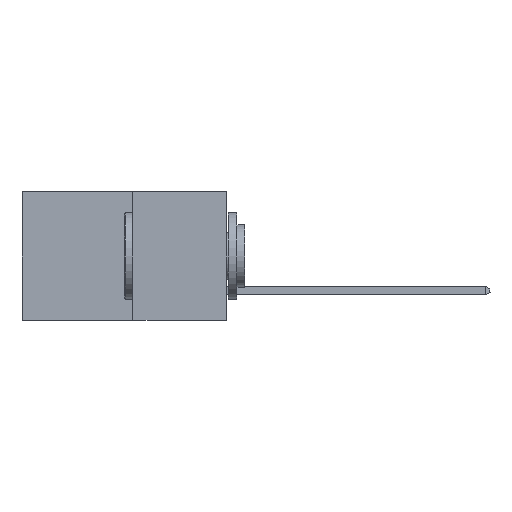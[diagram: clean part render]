
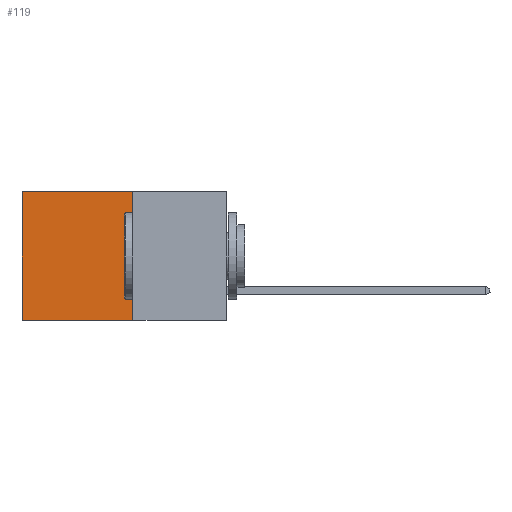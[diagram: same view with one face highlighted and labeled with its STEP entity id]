
A CAD part, left-side view. The second image highlights one B-rep face of the part: STEP entity #119.
In plain terms, the highlighted planar face has unit normal (-1, 0, 0).
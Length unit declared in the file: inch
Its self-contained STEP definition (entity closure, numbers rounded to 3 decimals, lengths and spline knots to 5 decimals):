
#119 = ADVANCED_FACE ( 'NONE', ( #27254 ), #26130, .F. ) ;
#1892 = DIRECTION ( 'NONE',  ( 1., 0., 0. ) ) ;
#3809 = DIRECTION ( 'NONE',  ( 0., 0., -1. ) ) ;
#4090 = EDGE_CURVE ( 'NONE', #14034, #9654, #15876, .T. ) ;
#4348 = ORIENTED_EDGE ( 'NONE', *, *, #4090, .T. ) ;
#4952 = CARTESIAN_POINT ( 'NONE',  ( 0.277, 0.59, 0. ) ) ;
#5809 = DIRECTION ( 'NONE',  ( 0., 1., 0. ) ) ;
#8598 = CARTESIAN_POINT ( 'NONE',  ( 0.277, 0.27, -0.37 ) ) ;
#8770 = VERTEX_POINT ( 'NONE', #8598 ) ;
#9345 = ORIENTED_EDGE ( 'NONE', *, *, #20863, .F. ) ;
#9654 = VERTEX_POINT ( 'NONE', #18343 ) ;
#9791 = DIRECTION ( 'NONE',  ( 0., 0., -1. ) ) ;
#9845 = CARTESIAN_POINT ( 'NONE',  ( 0.277, 0.27, 0. ) ) ;
#10617 = VECTOR ( 'NONE', #9791, 39.37008 ) ;
#12073 = CARTESIAN_POINT ( 'NONE',  ( 0.277, 0.27, 0. ) ) ;
#12479 = LINE ( 'NONE', #9845, #17585 ) ;
#13089 = ORIENTED_EDGE ( 'NONE', *, *, #24280, .F. ) ;
#14034 = VERTEX_POINT ( 'NONE', #4952 ) ;
#14149 = DIRECTION ( 'NONE',  ( 0., 1., 0. ) ) ;
#14561 = VECTOR ( 'NONE', #5809, 39.37008 ) ;
#15876 = LINE ( 'NONE', #24438, #26020 ) ;
#16377 = CARTESIAN_POINT ( 'NONE',  ( 0.277, 0.27, -0.37 ) ) ;
#16980 = CARTESIAN_POINT ( 'NONE',  ( 0.277, 0.27, -0.37 ) ) ;
#17585 = VECTOR ( 'NONE', #14149, 39.37008 ) ;
#18139 = VERTEX_POINT ( 'NONE', #12073 ) ;
#18343 = CARTESIAN_POINT ( 'NONE',  ( 0.277, 0.59, -0.37 ) ) ;
#18514 = EDGE_LOOP ( 'NONE', ( #4348, #13089, #9345, #23989 ) ) ;
#20352 = LINE ( 'NONE', #23153, #14561 ) ;
#20863 = EDGE_CURVE ( 'NONE', #18139, #8770, #27896, .T. ) ;
#20911 = AXIS2_PLACEMENT_3D ( 'NONE', #16980, #1892, #3809 ) ;
#23153 = CARTESIAN_POINT ( 'NONE',  ( 0.277, 0.27, -0.37 ) ) ;
#23989 = ORIENTED_EDGE ( 'NONE', *, *, #24851, .T. ) ;
#24091 = DIRECTION ( 'NONE',  ( 0., 0., -1. ) ) ;
#24280 = EDGE_CURVE ( 'NONE', #8770, #9654, #20352, .T. ) ;
#24438 = CARTESIAN_POINT ( 'NONE',  ( 0.277, 0.59, -0.37 ) ) ;
#24851 = EDGE_CURVE ( 'NONE', #18139, #14034, #12479, .T. ) ;
#26020 = VECTOR ( 'NONE', #24091, 39.37008 ) ;
#26130 = PLANE ( 'NONE',  #20911 ) ;
#27254 = FACE_OUTER_BOUND ( 'NONE', #18514, .T. ) ;
#27896 = LINE ( 'NONE', #16377, #10617 ) ;
